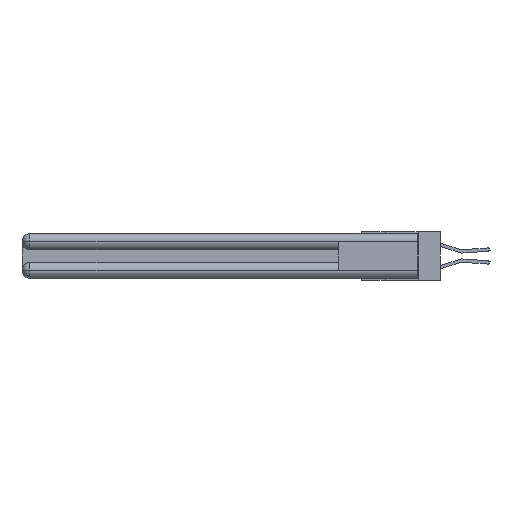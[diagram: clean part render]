
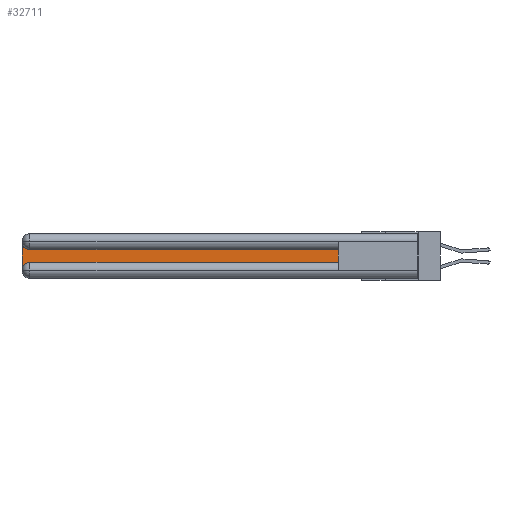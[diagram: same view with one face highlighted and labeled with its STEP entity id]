
A CAD part, left-side view. The second image highlights one B-rep face of the part: STEP entity #32711.
In plain terms, the highlighted planar face has unit normal (-1, 0, 0).
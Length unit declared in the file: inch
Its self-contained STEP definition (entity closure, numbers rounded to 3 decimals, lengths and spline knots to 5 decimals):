
#799 = CARTESIAN_POINT ( 'NONE',  ( 0.075, 2.94, -0.1225 ) ) ;
#823 = DIRECTION ( 'NONE',  ( 0., 0., -1. ) ) ;
#2649 = AXIS2_PLACEMENT_3D ( 'NONE', #23175, #7759, #30398 ) ;
#2761 = VERTEX_POINT ( 'NONE', #799 ) ;
#2921 = CARTESIAN_POINT ( 'NONE',  ( 0.075, 2.94, -0.2175 ) ) ;
#3545 = ORIENTED_EDGE ( 'NONE', *, *, #11709, .T. ) ;
#3679 = PLANE ( 'NONE',  #6222 ) ;
#4438 = CARTESIAN_POINT ( 'NONE',  ( 0.075, 3., -0.2775 ) ) ;
#4647 = DIRECTION ( 'NONE',  ( 0., 0., -1. ) ) ;
#5462 = LINE ( 'NONE', #25178, #22949 ) ;
#6222 = AXIS2_PLACEMENT_3D ( 'NONE', #21440, #26544, #29209 ) ;
#7402 = VECTOR ( 'NONE', #30616, 39.37008 ) ;
#7759 = DIRECTION ( 'NONE',  ( 1., 0., 0. ) ) ;
#8136 = CARTESIAN_POINT ( 'NONE',  ( 0.075, 0.6, -0.1225 ) ) ;
#8810 = CARTESIAN_POINT ( 'NONE',  ( 0.075, 3., -0.2175 ) ) ;
#9074 = ORIENTED_EDGE ( 'NONE', *, *, #16745, .T. ) ;
#9978 = DIRECTION ( 'NONE',  ( 0., -1., 0. ) ) ;
#10284 = CARTESIAN_POINT ( 'NONE',  ( 0.075, 0.6, -0.2175 ) ) ;
#11709 = EDGE_CURVE ( 'NONE', #14590, #21801, #17749, .T. ) ;
#12273 = CIRCLE ( 'NONE', #17415, 0.06 ) ;
#13067 = ORIENTED_EDGE ( 'NONE', *, *, #27708, .T. ) ;
#14590 = VERTEX_POINT ( 'NONE', #4438 ) ;
#14614 = FACE_OUTER_BOUND ( 'NONE', #28636, .T. ) ;
#16683 = ORIENTED_EDGE ( 'NONE', *, *, #18491, .T. ) ;
#16745 = EDGE_CURVE ( 'NONE', #24868, #2761, #28200, .T. ) ;
#17415 = AXIS2_PLACEMENT_3D ( 'NONE', #32314, #24960, #4647 ) ;
#17741 = EDGE_CURVE ( 'NONE', #21801, #20044, #5462, .T. ) ;
#17749 = CIRCLE ( 'NONE', #2649, 0.06 ) ;
#18491 = EDGE_CURVE ( 'NONE', #20044, #24868, #24871, .T. ) ;
#19977 = CARTESIAN_POINT ( 'NONE',  ( 0.075, 3., -0.0625 ) ) ;
#20044 = VERTEX_POINT ( 'NONE', #32606 ) ;
#21440 = CARTESIAN_POINT ( 'NONE',  ( 0.075, 3., -0.1225 ) ) ;
#21801 = VERTEX_POINT ( 'NONE', #2921 ) ;
#21928 = LINE ( 'NONE', #8810, #31106 ) ;
#22949 = VECTOR ( 'NONE', #9978, 39.37008 ) ;
#23175 = CARTESIAN_POINT ( 'NONE',  ( 0.075, 2.94, -0.2775 ) ) ;
#23465 = ORIENTED_EDGE ( 'NONE', *, *, #17741, .T. ) ;
#24868 = VERTEX_POINT ( 'NONE', #8136 ) ;
#24871 = LINE ( 'NONE', #10284, #7402 ) ;
#24960 = DIRECTION ( 'NONE',  ( 1., 0., 0. ) ) ;
#25178 = CARTESIAN_POINT ( 'NONE',  ( 0.075, 0.6, -0.2175 ) ) ;
#25374 = CARTESIAN_POINT ( 'NONE',  ( 0.075, 0.6, -0.1225 ) ) ;
#25723 = EDGE_CURVE ( 'NONE', #28307, #14590, #21928, .T. ) ;
#25893 = ORIENTED_EDGE ( 'NONE', *, *, #25723, .T. ) ;
#26544 = DIRECTION ( 'NONE',  ( 1., 0., 0. ) ) ;
#27708 = EDGE_CURVE ( 'NONE', #2761, #28307, #12273, .T. ) ;
#28200 = LINE ( 'NONE', #25374, #30579 ) ;
#28307 = VERTEX_POINT ( 'NONE', #19977 ) ;
#28636 = EDGE_LOOP ( 'NONE', ( #9074, #13067, #25893, #3545, #23465, #16683 ) ) ;
#29209 = DIRECTION ( 'NONE',  ( 0., 0., -1. ) ) ;
#30398 = DIRECTION ( 'NONE',  ( 0., 0., -1. ) ) ;
#30579 = VECTOR ( 'NONE', #30608, 39.37008 ) ;
#30608 = DIRECTION ( 'NONE',  ( 0., 1., 0. ) ) ;
#30616 = DIRECTION ( 'NONE',  ( 0., 0., 1. ) ) ;
#31106 = VECTOR ( 'NONE', #823, 39.37008 ) ;
#32314 = CARTESIAN_POINT ( 'NONE',  ( 0.075, 2.94, -0.0625 ) ) ;
#32606 = CARTESIAN_POINT ( 'NONE',  ( 0.075, 0.6, -0.2175 ) ) ;
#32711 = ADVANCED_FACE ( 'NONE', ( #14614 ), #3679, .F. ) ;
